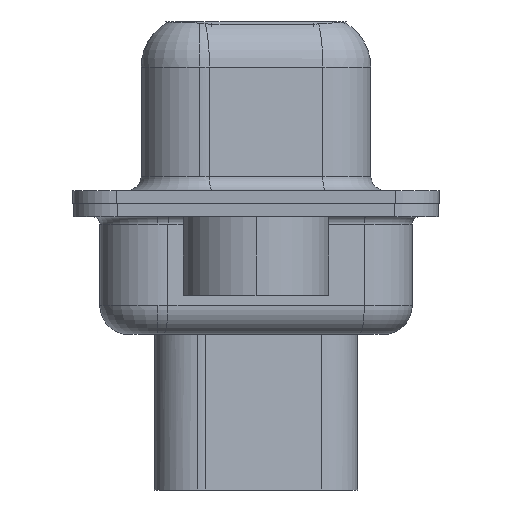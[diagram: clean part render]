
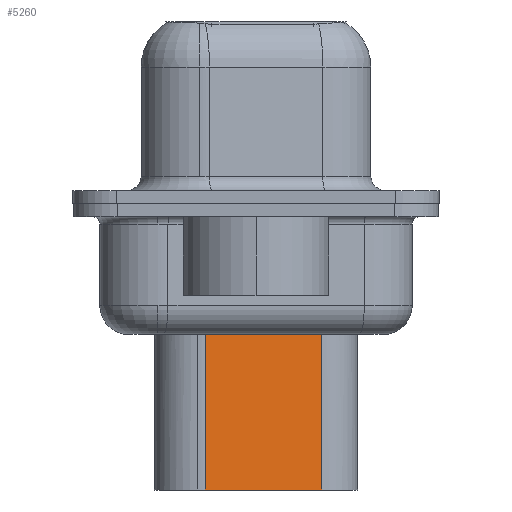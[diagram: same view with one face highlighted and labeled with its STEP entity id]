
A CAD part, left-side view. The second image highlights one B-rep face of the part: STEP entity #5260.
In plain terms, the highlighted planar face has unit normal (-0.985, -0.174, 0).
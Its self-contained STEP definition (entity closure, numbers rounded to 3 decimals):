
#925 = VERTEX_POINT ( 'NONE', #10028 ) ;
#981 = CARTESIAN_POINT ( 'NONE',  ( 5.214, -2.26, -9.85 ) ) ;
#1031 = ORIENTED_EDGE ( 'NONE', *, *, #2097, .F. ) ;
#1262 = VERTEX_POINT ( 'NONE', #981 ) ;
#1914 = DIRECTION ( 'NONE',  ( -0.174, 0.985, 0. ) ) ;
#2097 = EDGE_CURVE ( 'NONE', #9868, #1262, #18410, .T. ) ;
#2185 = LINE ( 'NONE', #7981, #4593 ) ;
#3581 = VECTOR ( 'NONE', #7558, 1000. ) ;
#4218 = DIRECTION ( 'NONE',  ( -0.985, -0.174, 0. ) ) ;
#4593 = VECTOR ( 'NONE', #16836, 1000. ) ;
#5038 = EDGE_CURVE ( 'NONE', #9868, #17437, #11761, .T. ) ;
#5260 = ADVANCED_FACE ( 'NONE', ( #6885 ), #14117, .T. ) ;
#6885 = FACE_OUTER_BOUND ( 'NONE', #10892, .T. ) ;
#7473 = CARTESIAN_POINT ( 'NONE',  ( 4.509, 1.74, -3.975 ) ) ;
#7558 = DIRECTION ( 'NONE',  ( -0.174, 0.985, 0. ) ) ;
#7981 = CARTESIAN_POINT ( 'NONE',  ( 4.509, 1.74, -3.1 ) ) ;
#8688 = CARTESIAN_POINT ( 'NONE',  ( 4.509, 1.74, -3.1 ) ) ;
#8775 = CARTESIAN_POINT ( 'NONE',  ( 4.509, 1.74, -9.85 ) ) ;
#8997 = CARTESIAN_POINT ( 'NONE',  ( 4.338, 2.709, -3.975 ) ) ;
#9466 = CARTESIAN_POINT ( 'NONE',  ( 5.214, -2.26, -3.1 ) ) ;
#9868 = VERTEX_POINT ( 'NONE', #10376 ) ;
#9881 = VECTOR ( 'NONE', #1914, 1000. ) ;
#10028 = CARTESIAN_POINT ( 'NONE',  ( 4.509, 1.74, -9.85 ) ) ;
#10376 = CARTESIAN_POINT ( 'NONE',  ( 5.214, -2.26, -3.975 ) ) ;
#10875 = VECTOR ( 'NONE', #16997, 1000. ) ;
#10892 = EDGE_LOOP ( 'NONE', ( #1031, #16439, #16416, #18494 ) ) ;
#11761 = LINE ( 'NONE', #8997, #3581 ) ;
#11850 = EDGE_CURVE ( 'NONE', #17437, #925, #2185, .T. ) ;
#14117 = PLANE ( 'NONE',  #14743 ) ;
#14682 = EDGE_CURVE ( 'NONE', #1262, #925, #16280, .T. ) ;
#14743 = AXIS2_PLACEMENT_3D ( 'NONE', #8688, #4218, #15546 ) ;
#15546 = DIRECTION ( 'NONE',  ( 0.174, -0.985, 0. ) ) ;
#16280 = LINE ( 'NONE', #8775, #9881 ) ;
#16416 = ORIENTED_EDGE ( 'NONE', *, *, #11850, .T. ) ;
#16439 = ORIENTED_EDGE ( 'NONE', *, *, #5038, .T. ) ;
#16836 = DIRECTION ( 'NONE',  ( 0., 0., -1. ) ) ;
#16997 = DIRECTION ( 'NONE',  ( 0., 0., -1. ) ) ;
#17437 = VERTEX_POINT ( 'NONE', #7473 ) ;
#18410 = LINE ( 'NONE', #9466, #10875 ) ;
#18494 = ORIENTED_EDGE ( 'NONE', *, *, #14682, .F. ) ;
